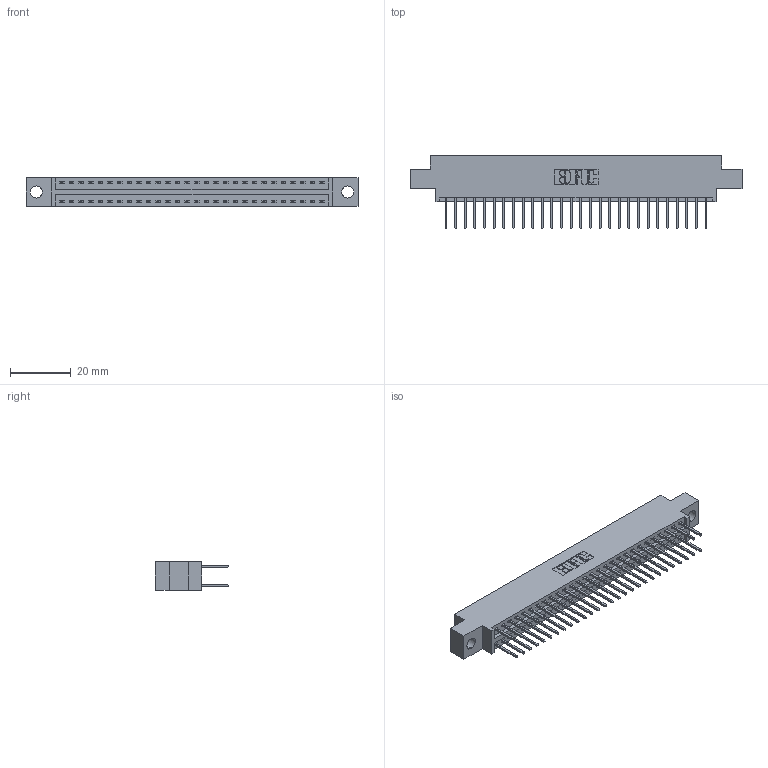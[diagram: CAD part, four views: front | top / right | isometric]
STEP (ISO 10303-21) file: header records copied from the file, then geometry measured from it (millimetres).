
FILE_DESCRIPTION (( 'STEP AP203' ), '1' );
FILE_NAME ('346-056-526-804.STEP', '2022-05-21T05:42:17', ( '' ), ( '' ), 'SwSTEP 2.0', 'SolidWorks 2020', '' );
FILE_SCHEMA (( 'CONFIG_CONTROL_DESIGN' ));
Length unit declared in the file: inch
Products named in the file (3): 346-056-526-804; 345-292-001_345-293-126; 346 Part_0.170 Offset - 0.156 Dia-TH
Assembly tree (57 placements, depth 2):
  346-056-526-804
    346 Part_0.170 Offset - 0.156 Dia-TH
    345-292-001_345-293-126  x56
Bounding box: 109.47 x 24.13 x 9.4 mm (x, y, z)
Volume: 10397.6 mm3; surface area: 14510.7 mm2
Topology: 57 solids, 57 shells, 3052 faces, 9057 edges, 5962 vertices
Faces by surface type: plane 2054, cylinder 998
Entity records: 20727 total; most frequent: CARTESIAN_POINT 3442, ORIENTED_EDGE 3374, DIRECTION 3083, EDGE_CURVE 1687, VECTOR 1443, LINE 1443, VERTEX_POINT 1122, AXIS2_PLACEMENT_3D 820
